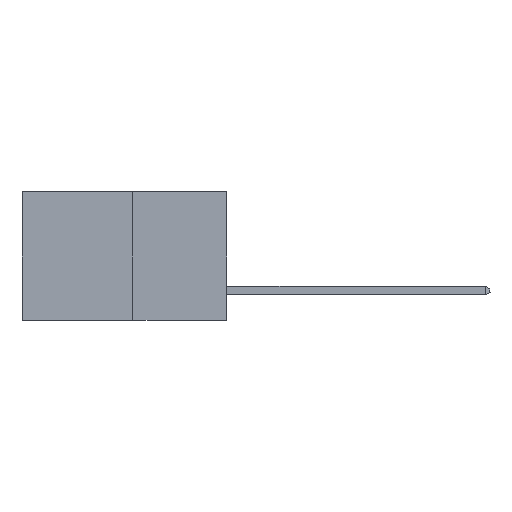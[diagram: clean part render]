
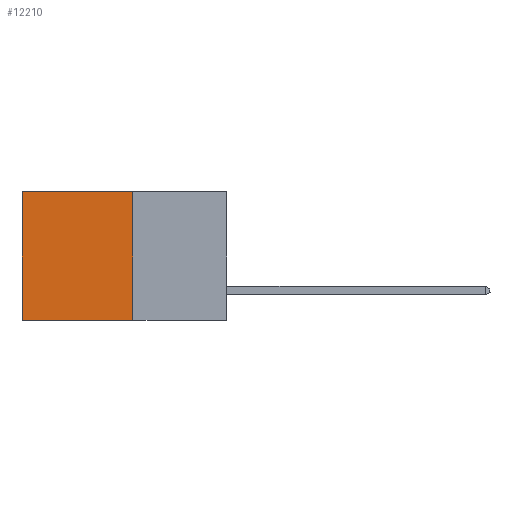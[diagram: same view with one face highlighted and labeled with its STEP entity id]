
A CAD part, left-side view. The second image highlights one B-rep face of the part: STEP entity #12210.
In plain terms, the highlighted planar face has unit normal (-1, 0, 0).
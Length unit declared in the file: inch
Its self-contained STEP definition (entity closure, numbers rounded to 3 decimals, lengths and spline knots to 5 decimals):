
#272 = VERTEX_POINT ( 'NONE', #2451 ) ;
#405 = CARTESIAN_POINT ( 'NONE',  ( 0.277, 0.59, -0.37 ) ) ;
#862 = EDGE_CURVE ( 'NONE', #272, #4873, #15703, .T. ) ;
#923 = EDGE_LOOP ( 'NONE', ( #8038, #15438, #7418, #10867 ) ) ;
#1736 = CARTESIAN_POINT ( 'NONE',  ( 0.277, 0.27, 0. ) ) ;
#2451 = CARTESIAN_POINT ( 'NONE',  ( 0.277, 0.27, -0.37 ) ) ;
#3100 = CARTESIAN_POINT ( 'NONE',  ( 0.277, 0.27, -0.37 ) ) ;
#3202 = VECTOR ( 'NONE', #10893, 39.37008 ) ;
#3241 = VECTOR ( 'NONE', #11800, 39.37008 ) ;
#3610 = DIRECTION ( 'NONE',  ( 1., 0., 0. ) ) ;
#4500 = CARTESIAN_POINT ( 'NONE',  ( 0.277, 0.59, 0. ) ) ;
#4873 = VERTEX_POINT ( 'NONE', #9888 ) ;
#5396 = VERTEX_POINT ( 'NONE', #4500 ) ;
#6422 = EDGE_CURVE ( 'NONE', #14286, #5396, #13547, .T. ) ;
#6437 = EDGE_CURVE ( 'NONE', #5396, #4873, #13150, .T. ) ;
#7274 = DIRECTION ( 'NONE',  ( 0., 0., -1. ) ) ;
#7418 = ORIENTED_EDGE ( 'NONE', *, *, #8232, .F. ) ;
#8038 = ORIENTED_EDGE ( 'NONE', *, *, #6437, .T. ) ;
#8232 = EDGE_CURVE ( 'NONE', #14286, #272, #10522, .T. ) ;
#8757 = CARTESIAN_POINT ( 'NONE',  ( 0.277, 0.27, -0.37 ) ) ;
#9582 = CARTESIAN_POINT ( 'NONE',  ( 0.277, 0.27, 0. ) ) ;
#9749 = VECTOR ( 'NONE', #7274, 39.37008 ) ;
#9888 = CARTESIAN_POINT ( 'NONE',  ( 0.277, 0.59, -0.37 ) ) ;
#10522 = LINE ( 'NONE', #3100, #3202 ) ;
#10863 = CARTESIAN_POINT ( 'NONE',  ( 0.277, 0.27, -0.37 ) ) ;
#10867 = ORIENTED_EDGE ( 'NONE', *, *, #6422, .T. ) ;
#10893 = DIRECTION ( 'NONE',  ( 0., 0., -1. ) ) ;
#11413 = PLANE ( 'NONE',  #12702 ) ;
#11800 = DIRECTION ( 'NONE',  ( 0., 1., 0. ) ) ;
#12210 = ADVANCED_FACE ( 'NONE', ( #15767 ), #11413, .F. ) ;
#12684 = DIRECTION ( 'NONE',  ( 0., 0., -1. ) ) ;
#12702 = AXIS2_PLACEMENT_3D ( 'NONE', #8757, #3610, #12684 ) ;
#12752 = VECTOR ( 'NONE', #16185, 39.37008 ) ;
#13150 = LINE ( 'NONE', #405, #9749 ) ;
#13547 = LINE ( 'NONE', #1736, #3241 ) ;
#14286 = VERTEX_POINT ( 'NONE', #9582 ) ;
#15438 = ORIENTED_EDGE ( 'NONE', *, *, #862, .F. ) ;
#15703 = LINE ( 'NONE', #10863, #12752 ) ;
#15767 = FACE_OUTER_BOUND ( 'NONE', #923, .T. ) ;
#16185 = DIRECTION ( 'NONE',  ( 0., 1., 0. ) ) ;
